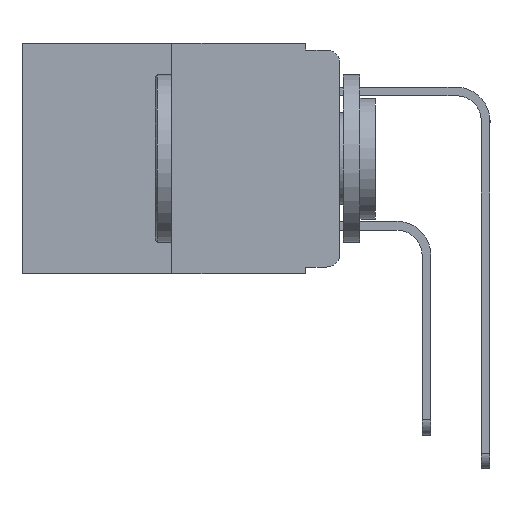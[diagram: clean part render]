
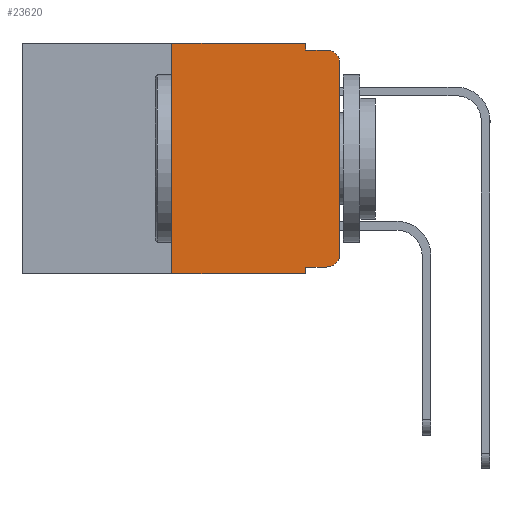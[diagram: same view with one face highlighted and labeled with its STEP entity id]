
A CAD part, left-side view. The second image highlights one B-rep face of the part: STEP entity #23620.
In plain terms, the highlighted planar face has unit normal (-1, 0, 0).
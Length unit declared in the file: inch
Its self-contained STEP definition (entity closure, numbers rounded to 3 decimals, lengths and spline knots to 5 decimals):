
#193 = CARTESIAN_POINT ( 'NONE',  ( 0., 0.051, -0.343 ) ) ;
#201 = VERTEX_POINT ( 'NONE', #12371 ) ;
#656 = LINE ( 'NONE', #11695, #13708 ) ;
#731 = DIRECTION ( 'NONE',  ( 0., 0., -1. ) ) ;
#815 = ORIENTED_EDGE ( 'NONE', *, *, #17325, .T. ) ;
#972 = VERTEX_POINT ( 'NONE', #193 ) ;
#1959 = LINE ( 'NONE', #10024, #4599 ) ;
#2198 = CARTESIAN_POINT ( 'NONE',  ( 0., 0.473, 0. ) ) ;
#3197 = VERTEX_POINT ( 'NONE', #13334 ) ;
#3383 = CIRCLE ( 'NONE', #8844, 0.02 ) ;
#3647 = EDGE_CURVE ( 'NONE', #12812, #16863, #3383, .T. ) ;
#3674 = LINE ( 'NONE', #21666, #23097 ) ;
#3702 = PLANE ( 'NONE',  #11131 ) ;
#3749 = CARTESIAN_POINT ( 'NONE',  ( 0., 0., 0. ) ) ;
#4535 = VERTEX_POINT ( 'NONE', #21920 ) ;
#4599 = VECTOR ( 'NONE', #20932, 39.37008 ) ;
#5143 = DIRECTION ( 'NONE',  ( 0., -1., 0. ) ) ;
#5243 = DIRECTION ( 'NONE',  ( 0., -1., 0. ) ) ;
#5460 = ORIENTED_EDGE ( 'NONE', *, *, #11547, .F. ) ;
#5535 = VECTOR ( 'NONE', #18754, 39.37008 ) ;
#5973 = LINE ( 'NONE', #3749, #16284 ) ;
#6116 = LINE ( 'NONE', #2198, #5535 ) ;
#6171 = CIRCLE ( 'NONE', #8282, 0.02 ) ;
#7019 = DIRECTION ( 'NONE',  ( 0., 0., -1. ) ) ;
#7040 = EDGE_CURVE ( 'NONE', #9146, #20791, #14232, .T. ) ;
#7656 = VERTEX_POINT ( 'NONE', #8643 ) ;
#7780 = VECTOR ( 'NONE', #731, 39.37008 ) ;
#8270 = EDGE_CURVE ( 'NONE', #8508, #4535, #6116, .T. ) ;
#8282 = AXIS2_PLACEMENT_3D ( 'NONE', #21797, #10928, #23625 ) ;
#8508 = VERTEX_POINT ( 'NONE', #15718 ) ;
#8542 = CARTESIAN_POINT ( 'NONE',  ( 0., 0.051, -0.333 ) ) ;
#8643 = CARTESIAN_POINT ( 'NONE',  ( 0., 0.051, -0.01 ) ) ;
#8844 = AXIS2_PLACEMENT_3D ( 'NONE', #23352, #23112, #7019 ) ;
#9146 = VERTEX_POINT ( 'NONE', #8542 ) ;
#9258 = DIRECTION ( 'NONE',  ( 1., 0., 0. ) ) ;
#10024 = CARTESIAN_POINT ( 'NONE',  ( 0., 0.25, 0. ) ) ;
#10928 = DIRECTION ( 'NONE',  ( -1., 0., 0. ) ) ;
#11041 = CARTESIAN_POINT ( 'NONE',  ( 0., 0.473, 0. ) ) ;
#11131 = AXIS2_PLACEMENT_3D ( 'NONE', #11041, #9258, #21992 ) ;
#11501 = VECTOR ( 'NONE', #11553, 39.37008 ) ;
#11547 = EDGE_CURVE ( 'NONE', #4535, #7656, #17513, .T. ) ;
#11553 = DIRECTION ( 'NONE',  ( 0., 0., -1. ) ) ;
#11695 = CARTESIAN_POINT ( 'NONE',  ( 0., 0.473, -0.343 ) ) ;
#11801 = ORIENTED_EDGE ( 'NONE', *, *, #3647, .T. ) ;
#12371 = CARTESIAN_POINT ( 'NONE',  ( 0., 0.25, -0.343 ) ) ;
#12812 = VERTEX_POINT ( 'NONE', #15784 ) ;
#13239 = EDGE_CURVE ( 'NONE', #9146, #972, #16340, .T. ) ;
#13257 = ORIENTED_EDGE ( 'NONE', *, *, #8270, .F. ) ;
#13334 = CARTESIAN_POINT ( 'NONE',  ( 0., 0., -0.313 ) ) ;
#13530 = DIRECTION ( 'NONE',  ( 0., -1., 0. ) ) ;
#13708 = VECTOR ( 'NONE', #13530, 39.37008 ) ;
#14232 = LINE ( 'NONE', #17949, #18497 ) ;
#14951 = EDGE_CURVE ( 'NONE', #201, #972, #656, .T. ) ;
#14991 = ORIENTED_EDGE ( 'NONE', *, *, #13239, .F. ) ;
#15718 = CARTESIAN_POINT ( 'NONE',  ( 0., 0.25, 0. ) ) ;
#15784 = CARTESIAN_POINT ( 'NONE',  ( 0., 0., -0.03 ) ) ;
#16284 = VECTOR ( 'NONE', #16617, 39.37008 ) ;
#16340 = LINE ( 'NONE', #20600, #11501 ) ;
#16617 = DIRECTION ( 'NONE',  ( 0., 0., 1. ) ) ;
#16863 = VERTEX_POINT ( 'NONE', #20956 ) ;
#17223 = ORIENTED_EDGE ( 'NONE', *, *, #20515, .F. ) ;
#17325 = EDGE_CURVE ( 'NONE', #20791, #3197, #6171, .T. ) ;
#17513 = LINE ( 'NONE', #20894, #7780 ) ;
#17949 = CARTESIAN_POINT ( 'NONE',  ( 0., 0.051, -0.333 ) ) ;
#17983 = EDGE_LOOP ( 'NONE', ( #20311, #11801, #23700, #5460, #13257, #17223, #21182, #14991, #22617, #815 ) ) ;
#18497 = VECTOR ( 'NONE', #5143, 39.37008 ) ;
#18562 = FACE_OUTER_BOUND ( 'NONE', #17983, .T. ) ;
#18754 = DIRECTION ( 'NONE',  ( 0., -1., 0. ) ) ;
#20311 = ORIENTED_EDGE ( 'NONE', *, *, #22022, .T. ) ;
#20515 = EDGE_CURVE ( 'NONE', #201, #8508, #1959, .T. ) ;
#20600 = CARTESIAN_POINT ( 'NONE',  ( 0., 0.051, 0. ) ) ;
#20791 = VERTEX_POINT ( 'NONE', #23360 ) ;
#20894 = CARTESIAN_POINT ( 'NONE',  ( 0., 0.051, 0. ) ) ;
#20932 = DIRECTION ( 'NONE',  ( 0., 0., 1. ) ) ;
#20956 = CARTESIAN_POINT ( 'NONE',  ( 0., 0.02, -0.01 ) ) ;
#21182 = ORIENTED_EDGE ( 'NONE', *, *, #14951, .T. ) ;
#21258 = EDGE_CURVE ( 'NONE', #7656, #16863, #3674, .T. ) ;
#21666 = CARTESIAN_POINT ( 'NONE',  ( 0., 0.051, -0.01 ) ) ;
#21797 = CARTESIAN_POINT ( 'NONE',  ( 0., 0.02, -0.313 ) ) ;
#21920 = CARTESIAN_POINT ( 'NONE',  ( 0., 0.051, 0. ) ) ;
#21992 = DIRECTION ( 'NONE',  ( 0., 0., -1. ) ) ;
#22022 = EDGE_CURVE ( 'NONE', #3197, #12812, #5973, .T. ) ;
#22617 = ORIENTED_EDGE ( 'NONE', *, *, #7040, .T. ) ;
#23097 = VECTOR ( 'NONE', #5243, 39.37008 ) ;
#23112 = DIRECTION ( 'NONE',  ( -1., 0., 0. ) ) ;
#23352 = CARTESIAN_POINT ( 'NONE',  ( 0., 0.02, -0.03 ) ) ;
#23360 = CARTESIAN_POINT ( 'NONE',  ( 0., 0.02, -0.333 ) ) ;
#23620 = ADVANCED_FACE ( 'NONE', ( #18562 ), #3702, .F. ) ;
#23625 = DIRECTION ( 'NONE',  ( 0., 0., -1. ) ) ;
#23700 = ORIENTED_EDGE ( 'NONE', *, *, #21258, .F. ) ;
